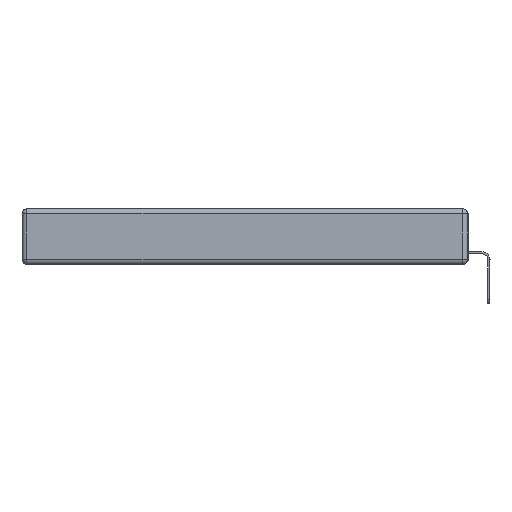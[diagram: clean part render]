
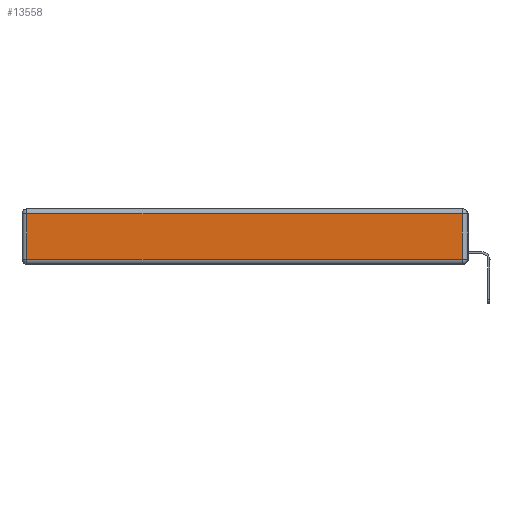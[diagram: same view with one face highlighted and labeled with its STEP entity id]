
A CAD part, left-side view. The second image highlights one B-rep face of the part: STEP entity #13558.
In plain terms, the highlighted planar face has unit normal (-1, 0, 0).
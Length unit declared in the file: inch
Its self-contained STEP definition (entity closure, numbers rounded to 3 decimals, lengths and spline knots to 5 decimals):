
#168 = LINE ( 'NONE', #5065, #10138 ) ;
#192 = DIRECTION ( 'NONE',  ( 0., 0., 1. ) ) ;
#751 = ORIENTED_EDGE ( 'NONE', *, *, #14977, .T. ) ;
#832 = CARTESIAN_POINT ( 'NONE',  ( 0., 0.03, -0.03 ) ) ;
#1419 = CARTESIAN_POINT ( 'NONE',  ( 0., 0., -0.343 ) ) ;
#2842 = VERTEX_POINT ( 'NONE', #9337 ) ;
#2868 = EDGE_CURVE ( 'NONE', #14073, #8004, #168, .T. ) ;
#3030 = EDGE_CURVE ( 'NONE', #2842, #14438, #15853, .T. ) ;
#5065 = CARTESIAN_POINT ( 'NONE',  ( 0., 2.72, -0.343 ) ) ;
#5792 = DIRECTION ( 'NONE',  ( -1., 0., 0. ) ) ;
#5987 = FACE_OUTER_BOUND ( 'NONE', #13733, .T. ) ;
#6552 = CARTESIAN_POINT ( 'NONE',  ( 0., 2.75, -0.03 ) ) ;
#6614 = ORIENTED_EDGE ( 'NONE', *, *, #3030, .T. ) ;
#7286 = LINE ( 'NONE', #6552, #14114 ) ;
#7910 = DIRECTION ( 'NONE',  ( 0., 0., -1. ) ) ;
#7929 = DIRECTION ( 'NONE',  ( 0., 1., 0. ) ) ;
#8004 = VERTEX_POINT ( 'NONE', #17236 ) ;
#8158 = DIRECTION ( 'NONE',  ( 0., 0., 1. ) ) ;
#8263 = EDGE_CURVE ( 'NONE', #8004, #2842, #17793, .T. ) ;
#8599 = PLANE ( 'NONE',  #14221 ) ;
#8923 = ORIENTED_EDGE ( 'NONE', *, *, #8263, .T. ) ;
#9337 = CARTESIAN_POINT ( 'NONE',  ( 0., 0.03, -0.313 ) ) ;
#10138 = VECTOR ( 'NONE', #7910, 39.37008 ) ;
#11066 = CARTESIAN_POINT ( 'NONE',  ( 0., 0., -0.313 ) ) ;
#11473 = VECTOR ( 'NONE', #8158, 39.37008 ) ;
#11510 = ORIENTED_EDGE ( 'NONE', *, *, #2868, .T. ) ;
#12479 = CARTESIAN_POINT ( 'NONE',  ( 0., 0.03, -0.343 ) ) ;
#13558 = ADVANCED_FACE ( 'NONE', ( #5987 ), #8599, .T. ) ;
#13733 = EDGE_LOOP ( 'NONE', ( #8923, #6614, #751, #11510 ) ) ;
#14026 = VECTOR ( 'NONE', #14985, 39.37008 ) ;
#14073 = VERTEX_POINT ( 'NONE', #15245 ) ;
#14114 = VECTOR ( 'NONE', #7929, 39.37008 ) ;
#14221 = AXIS2_PLACEMENT_3D ( 'NONE', #1419, #5792, #192 ) ;
#14438 = VERTEX_POINT ( 'NONE', #832 ) ;
#14977 = EDGE_CURVE ( 'NONE', #14438, #14073, #7286, .T. ) ;
#14985 = DIRECTION ( 'NONE',  ( 0., -1., 0. ) ) ;
#15245 = CARTESIAN_POINT ( 'NONE',  ( 0., 2.72, -0.03 ) ) ;
#15853 = LINE ( 'NONE', #12479, #11473 ) ;
#17236 = CARTESIAN_POINT ( 'NONE',  ( 0., 2.72, -0.313 ) ) ;
#17793 = LINE ( 'NONE', #11066, #14026 ) ;
